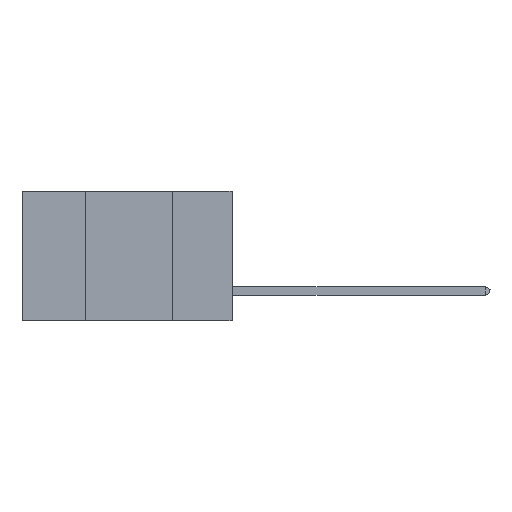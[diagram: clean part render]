
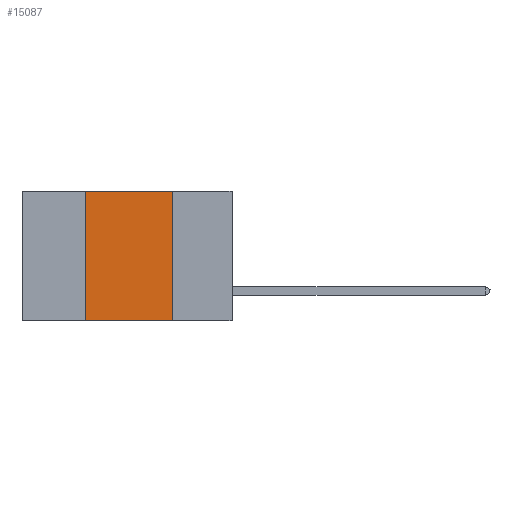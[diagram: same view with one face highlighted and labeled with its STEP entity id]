
A CAD part, left-side view. The second image highlights one B-rep face of the part: STEP entity #15087.
In plain terms, the highlighted planar face has unit normal (-1, 0, 0).
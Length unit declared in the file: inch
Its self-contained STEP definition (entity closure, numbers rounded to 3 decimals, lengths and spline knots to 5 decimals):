
#421 = LINE ( 'NONE', #14710, #13128 ) ;
#476 = CARTESIAN_POINT ( 'NONE',  ( 0., 0.6, 0. ) ) ;
#611 = VERTEX_POINT ( 'NONE', #12431 ) ;
#645 = LINE ( 'NONE', #10228, #11838 ) ;
#971 = DIRECTION ( 'NONE',  ( 0., 0., -1. ) ) ;
#1058 = VERTEX_POINT ( 'NONE', #16208 ) ;
#2249 = CARTESIAN_POINT ( 'NONE',  ( 0., 0.6, 0. ) ) ;
#2804 = EDGE_CURVE ( 'NONE', #7929, #611, #421, .T. ) ;
#3702 = LINE ( 'NONE', #6958, #10057 ) ;
#5048 = DIRECTION ( 'NONE',  ( 0., -1., 0. ) ) ;
#5917 = ORIENTED_EDGE ( 'NONE', *, *, #10109, .F. ) ;
#6958 = CARTESIAN_POINT ( 'NONE',  ( 0., 0.42, 0. ) ) ;
#7686 = ORIENTED_EDGE ( 'NONE', *, *, #2804, .T. ) ;
#7929 = VERTEX_POINT ( 'NONE', #11852 ) ;
#8848 = EDGE_CURVE ( 'NONE', #9681, #1058, #17580, .T. ) ;
#8873 = DIRECTION ( 'NONE',  ( 0., 0., -1. ) ) ;
#9003 = AXIS2_PLACEMENT_3D ( 'NONE', #2249, #9393, #971 ) ;
#9201 = EDGE_LOOP ( 'NONE', ( #5917, #16376, #16715, #7686 ) ) ;
#9216 = PLANE ( 'NONE',  #9003 ) ;
#9277 = VECTOR ( 'NONE', #11514, 39.37008 ) ;
#9393 = DIRECTION ( 'NONE',  ( 1., 0., 0. ) ) ;
#9681 = VERTEX_POINT ( 'NONE', #10665 ) ;
#10057 = VECTOR ( 'NONE', #14350, 39.37008 ) ;
#10109 = EDGE_CURVE ( 'NONE', #1058, #611, #645, .T. ) ;
#10228 = CARTESIAN_POINT ( 'NONE',  ( 0., 0.17, 0. ) ) ;
#10665 = CARTESIAN_POINT ( 'NONE',  ( 0., 0.42, 0. ) ) ;
#11098 = EDGE_CURVE ( 'NONE', #7929, #9681, #3702, .T. ) ;
#11514 = DIRECTION ( 'NONE',  ( 0., -1., 0. ) ) ;
#11838 = VECTOR ( 'NONE', #8873, 39.37008 ) ;
#11852 = CARTESIAN_POINT ( 'NONE',  ( 0., 0.42, -0.37 ) ) ;
#12431 = CARTESIAN_POINT ( 'NONE',  ( 0., 0.17, -0.37 ) ) ;
#13128 = VECTOR ( 'NONE', #5048, 39.37008 ) ;
#14350 = DIRECTION ( 'NONE',  ( 0., 0., 1. ) ) ;
#14710 = CARTESIAN_POINT ( 'NONE',  ( 0., 0.6, -0.37 ) ) ;
#15087 = ADVANCED_FACE ( 'NONE', ( #16449 ), #9216, .F. ) ;
#16208 = CARTESIAN_POINT ( 'NONE',  ( 0., 0.17, 0. ) ) ;
#16376 = ORIENTED_EDGE ( 'NONE', *, *, #8848, .F. ) ;
#16449 = FACE_OUTER_BOUND ( 'NONE', #9201, .T. ) ;
#16715 = ORIENTED_EDGE ( 'NONE', *, *, #11098, .F. ) ;
#17580 = LINE ( 'NONE', #476, #9277 ) ;
